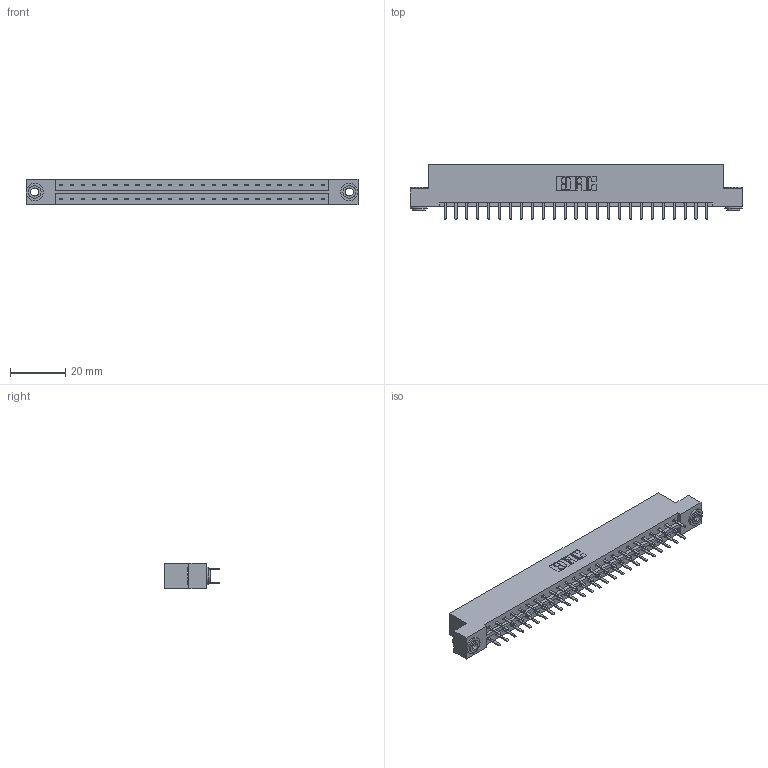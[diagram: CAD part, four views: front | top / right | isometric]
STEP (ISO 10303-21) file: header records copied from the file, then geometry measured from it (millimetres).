
FILE_DESCRIPTION (( 'STEP AP203' ), '1' );
FILE_NAME ('833-050-520-203.STEP', '2020-06-04T17:01:01', ( '' ), ( '' ), 'SwSTEP 2.0', 'SolidWorks 2020', '' );
FILE_SCHEMA (( 'CONFIG_CONTROL_DESIGN' ));
Length unit declared in the file: inch
Products named in the file (4): 345-250-002_345-250-002-102; 833 Part_Flush - .156 Dia - TH; 345-292-001_345-293-120; 833-050-520-203
Assembly tree (53 placements, depth 2):
  833-050-520-203
    833 Part_Flush - .156 Dia - TH
    345-292-001_345-293-120  x50
    345-250-002_345-250-002-102  x2
Bounding box: 120.6 x 20.02 x 9.4 mm (x, y, z)
Volume: 12150.9 mm3; surface area: 14345.4 mm2
Topology: 53 solids, 53 shells, 2952 faces, 8537 edges, 5554 vertices
Faces by surface type: plane 1980, cylinder 964, cone 8
Entity records: 19046 total; most frequent: CARTESIAN_POINT 3165, ORIENTED_EDGE 3082, DIRECTION 2755, EDGE_CURVE 1541, VECTOR 1385, LINE 1385, VERTEX_POINT 1022, AXIS2_PLACEMENT_3D 685
